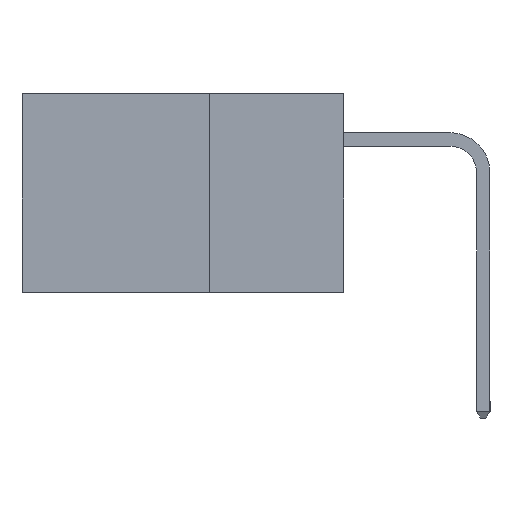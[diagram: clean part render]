
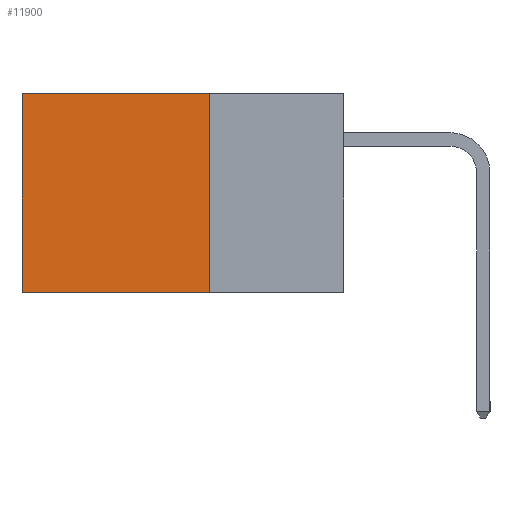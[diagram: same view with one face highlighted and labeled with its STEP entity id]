
A CAD part, left-side view. The second image highlights one B-rep face of the part: STEP entity #11900.
In plain terms, the highlighted planar face has unit normal (-1, 0, 0).
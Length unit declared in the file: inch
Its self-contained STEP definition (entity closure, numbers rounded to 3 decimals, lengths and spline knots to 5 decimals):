
#266 = PLANE ( 'NONE',  #8475 ) ;
#395 = VECTOR ( 'NONE', #4373, 39.37008 ) ;
#406 = EDGE_CURVE ( 'NONE', #12398, #16701, #10303, .T. ) ;
#783 = EDGE_LOOP ( 'NONE', ( #1160, #18793, #4853, #7402 ) ) ;
#1160 = ORIENTED_EDGE ( 'NONE', *, *, #17669, .T. ) ;
#1896 = DIRECTION ( 'NONE',  ( 0., 0., -1. ) ) ;
#2117 = CARTESIAN_POINT ( 'NONE',  ( 0.2615, 0.25, -0.37 ) ) ;
#2734 = CARTESIAN_POINT ( 'NONE',  ( 0.2615, 0.6, -0.37 ) ) ;
#2896 = CARTESIAN_POINT ( 'NONE',  ( 0.2615, 0.25, -0.37 ) ) ;
#4373 = DIRECTION ( 'NONE',  ( 0., 1., 0. ) ) ;
#4462 = CARTESIAN_POINT ( 'NONE',  ( 0.2615, 0.25, 0. ) ) ;
#4853 = ORIENTED_EDGE ( 'NONE', *, *, #406, .F. ) ;
#5540 = DIRECTION ( 'NONE',  ( 0., 0., -1. ) ) ;
#6219 = CARTESIAN_POINT ( 'NONE',  ( 0.2615, 0.25, -0.37 ) ) ;
#6261 = DIRECTION ( 'NONE',  ( 0., 0., -1. ) ) ;
#6279 = VECTOR ( 'NONE', #6822, 39.37008 ) ;
#6822 = DIRECTION ( 'NONE',  ( 0., 1., 0. ) ) ;
#7402 = ORIENTED_EDGE ( 'NONE', *, *, #14873, .T. ) ;
#7597 = LINE ( 'NONE', #8693, #11221 ) ;
#8475 = AXIS2_PLACEMENT_3D ( 'NONE', #15653, #11282, #1896 ) ;
#8693 = CARTESIAN_POINT ( 'NONE',  ( 0.2615, 0.6, -0.37 ) ) ;
#10303 = LINE ( 'NONE', #6219, #17684 ) ;
#11221 = VECTOR ( 'NONE', #5540, 39.37008 ) ;
#11282 = DIRECTION ( 'NONE',  ( 1., 0., 0. ) ) ;
#11683 = VERTEX_POINT ( 'NONE', #2734 ) ;
#11900 = ADVANCED_FACE ( 'NONE', ( #14656 ), #266, .F. ) ;
#12398 = VERTEX_POINT ( 'NONE', #4462 ) ;
#12914 = LINE ( 'NONE', #15136, #395 ) ;
#14451 = LINE ( 'NONE', #2117, #6279 ) ;
#14656 = FACE_OUTER_BOUND ( 'NONE', #783, .T. ) ;
#14873 = EDGE_CURVE ( 'NONE', #12398, #16800, #12914, .T. ) ;
#15136 = CARTESIAN_POINT ( 'NONE',  ( 0.2615, 0.25, 0. ) ) ;
#15484 = CARTESIAN_POINT ( 'NONE',  ( 0.2615, 0.6, 0. ) ) ;
#15653 = CARTESIAN_POINT ( 'NONE',  ( 0.2615, 0.25, -0.37 ) ) ;
#16701 = VERTEX_POINT ( 'NONE', #2896 ) ;
#16800 = VERTEX_POINT ( 'NONE', #15484 ) ;
#16990 = EDGE_CURVE ( 'NONE', #16701, #11683, #14451, .T. ) ;
#17669 = EDGE_CURVE ( 'NONE', #16800, #11683, #7597, .T. ) ;
#17684 = VECTOR ( 'NONE', #6261, 39.37008 ) ;
#18793 = ORIENTED_EDGE ( 'NONE', *, *, #16990, .F. ) ;
